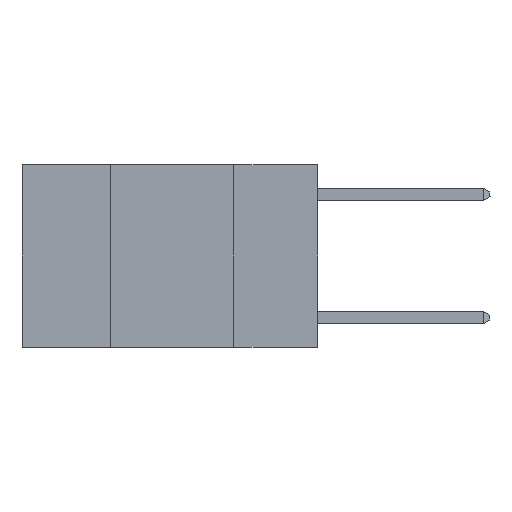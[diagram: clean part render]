
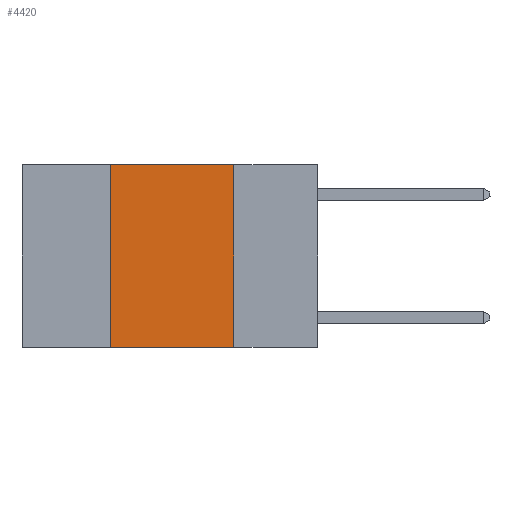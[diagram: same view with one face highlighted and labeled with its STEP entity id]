
A CAD part, left-side view. The second image highlights one B-rep face of the part: STEP entity #4420.
In plain terms, the highlighted planar face has unit normal (-1, 0, 0).
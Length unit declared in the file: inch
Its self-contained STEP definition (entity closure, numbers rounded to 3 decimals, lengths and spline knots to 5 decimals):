
#246 = CARTESIAN_POINT ( 'NONE',  ( 0., 0.6, 0. ) ) ;
#782 = EDGE_CURVE ( 'NONE', #9118, #5427, #2998, .T. ) ;
#930 = VECTOR ( 'NONE', #5713, 39.37008 ) ;
#1198 = VERTEX_POINT ( 'NONE', #5084 ) ;
#1594 = CARTESIAN_POINT ( 'NONE',  ( 0., 0.6, -0.37 ) ) ;
#2042 = LINE ( 'NONE', #2791, #7932 ) ;
#2206 = AXIS2_PLACEMENT_3D ( 'NONE', #3296, #8461, #4919 ) ;
#2791 = CARTESIAN_POINT ( 'NONE',  ( 0., 0.17, 0. ) ) ;
#2998 = LINE ( 'NONE', #8599, #930 ) ;
#3129 = VERTEX_POINT ( 'NONE', #8550 ) ;
#3296 = CARTESIAN_POINT ( 'NONE',  ( 0., 0.6, 0. ) ) ;
#3806 = FACE_OUTER_BOUND ( 'NONE', #4582, .T. ) ;
#4420 = ADVANCED_FACE ( 'NONE', ( #3806 ), #5626, .F. ) ;
#4437 = ORIENTED_EDGE ( 'NONE', *, *, #8737, .F. ) ;
#4582 = EDGE_LOOP ( 'NONE', ( #6383, #4437, #6931, #5615 ) ) ;
#4919 = DIRECTION ( 'NONE',  ( 0., 0., -1. ) ) ;
#5084 = CARTESIAN_POINT ( 'NONE',  ( 0., 0.17, 0. ) ) ;
#5335 = CARTESIAN_POINT ( 'NONE',  ( 0., 0.42, -0.37 ) ) ;
#5427 = VERTEX_POINT ( 'NONE', #5508 ) ;
#5508 = CARTESIAN_POINT ( 'NONE',  ( 0., 0.42, 0. ) ) ;
#5615 = ORIENTED_EDGE ( 'NONE', *, *, #9875, .T. ) ;
#5626 = PLANE ( 'NONE',  #2206 ) ;
#5642 = LINE ( 'NONE', #1594, #9466 ) ;
#5713 = DIRECTION ( 'NONE',  ( 0., 0., 1. ) ) ;
#6383 = ORIENTED_EDGE ( 'NONE', *, *, #8930, .F. ) ;
#6931 = ORIENTED_EDGE ( 'NONE', *, *, #782, .F. ) ;
#7744 = DIRECTION ( 'NONE',  ( 0., -1., 0. ) ) ;
#7932 = VECTOR ( 'NONE', #8154, 39.37008 ) ;
#8057 = LINE ( 'NONE', #246, #9372 ) ;
#8154 = DIRECTION ( 'NONE',  ( 0., 0., -1. ) ) ;
#8461 = DIRECTION ( 'NONE',  ( 1., 0., 0. ) ) ;
#8550 = CARTESIAN_POINT ( 'NONE',  ( 0., 0.17, -0.37 ) ) ;
#8599 = CARTESIAN_POINT ( 'NONE',  ( 0., 0.42, 0. ) ) ;
#8737 = EDGE_CURVE ( 'NONE', #5427, #1198, #8057, .T. ) ;
#8930 = EDGE_CURVE ( 'NONE', #1198, #3129, #2042, .T. ) ;
#9118 = VERTEX_POINT ( 'NONE', #5335 ) ;
#9372 = VECTOR ( 'NONE', #9461, 39.37008 ) ;
#9461 = DIRECTION ( 'NONE',  ( 0., -1., 0. ) ) ;
#9466 = VECTOR ( 'NONE', #7744, 39.37008 ) ;
#9875 = EDGE_CURVE ( 'NONE', #9118, #3129, #5642, .T. ) ;
